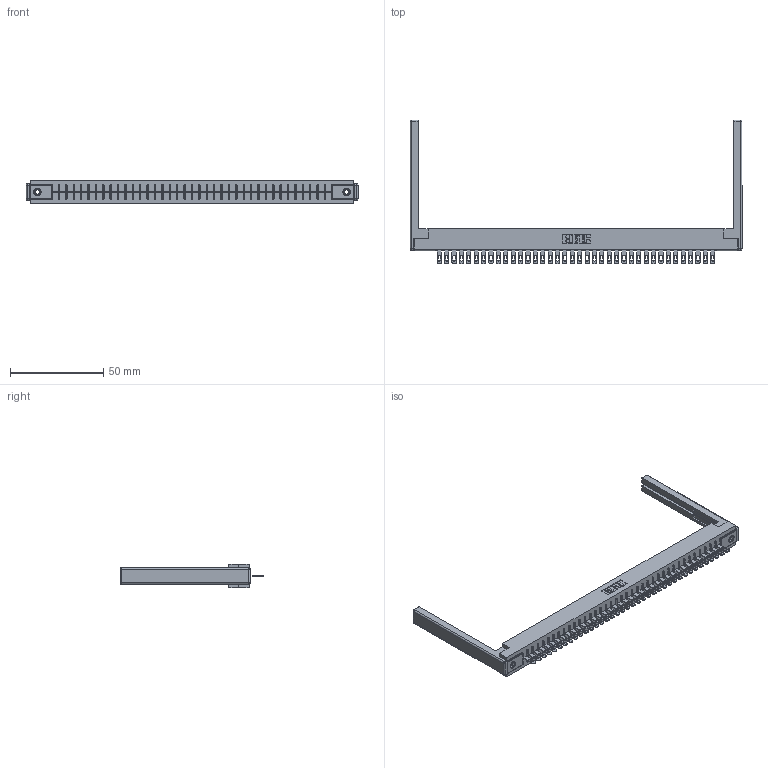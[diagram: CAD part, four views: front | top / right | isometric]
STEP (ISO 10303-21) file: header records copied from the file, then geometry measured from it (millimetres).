
FILE_DESCRIPTION (( 'STEP AP203' ), '1' );
FILE_NAME ('306-038-500-168.STEP', '2019-09-11T23:54:53', ( '' ), ( '' ), 'SwSTEP 2.0', 'SolidWorks 2016', '' );
FILE_SCHEMA (( 'CONFIG_CONTROL_DESIGN' ));
Length unit declared in the file: inch
Products named in the file (5): 307-220-068; 345-250-001_345-250-001-102; 306-038-500-168; 306-290-001_100; 306 Part_.156 Dia
Assembly tree (43 placements, depth 2):
  306-038-500-168
    306 Part_.156 Dia
    306-290-001_100  x38
    345-250-001_345-250-001-102  x2
    307-220-068  x2
Bounding box: 178 x 77.17 x 12.7 mm (x, y, z)
Volume: 24131.9 mm3; surface area: 24980.5 mm2
Topology: 43 solids, 43 shells, 3158 faces, 8876 edges, 5692 vertices
Faces by surface type: plane 2056, cylinder 926, sphere 160, cone 12, torus 4
Entity records: 38878 total; most frequent: CARTESIAN_POINT 6494, ORIENTED_EDGE 6430, DIRECTION 6417, EDGE_CURVE 3215, LINE 2507, VECTOR 2507, VERTEX_POINT 2032, AXIS2_PLACEMENT_3D 1955
